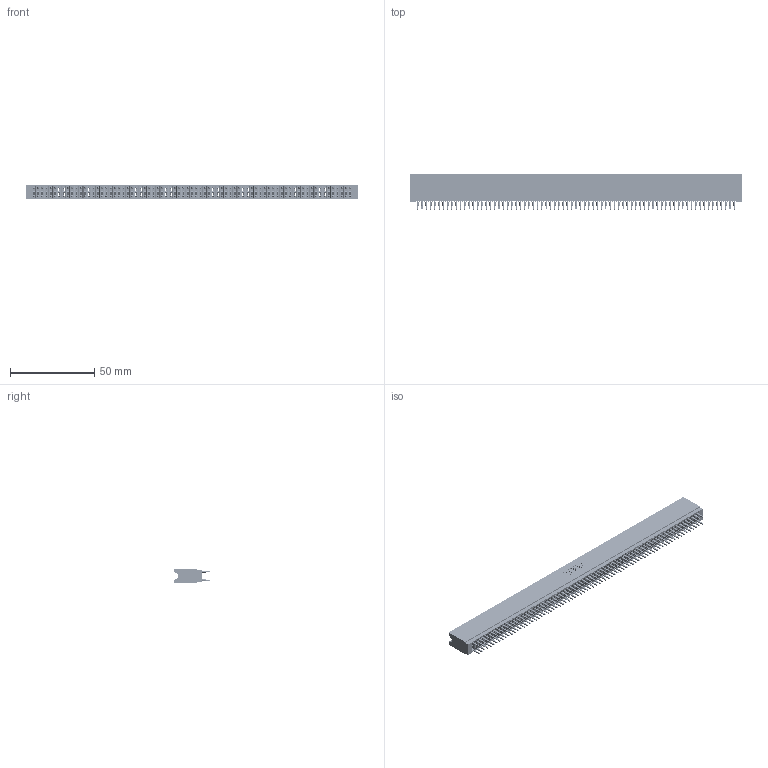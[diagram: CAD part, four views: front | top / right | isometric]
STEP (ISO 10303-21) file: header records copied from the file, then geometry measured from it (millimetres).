
FILE_DESCRIPTION (( 'STEP AP203' ), '1' );
FILE_NAME ('745-150-560-206.STEP', '2026-02-27T05:13:29', ( '' ), ( '' ), 'SwSTEP 2.0', 'SolidWorks 2023', '' );
FILE_SCHEMA (( 'CONFIG_CONTROL_DESIGN' ));
Products named in the file (3): 745 Part_Insulator Option - 06; 745-292-001_560; 745-150-560-206
Assembly tree (151 placements, depth 2):
  745-150-560-206
    745 Part_Insulator Option - 06
    745-292-001_560  x150
Bounding box: 197.1 x 21.22 x 8.89 mm (x, y, z)
Volume: 18083.5 mm3; surface area: 39919.7 mm2
Topology: 151 solids, 151 shells, 14871 faces, 40685 edges, 25822 vertices
Faces by surface type: plane 7706, cylinder 3265, bspline 3000, torus 900
Entity records: 122102 total; most frequent: CARTESIAN_POINT 21672, ORIENTED_EDGE 21174, DIRECTION 18473, EDGE_CURVE 10587, VECTOR 9947, LINE 9947, VERTEX_POINT 6750, AXIS2_PLACEMENT_3D 4263
